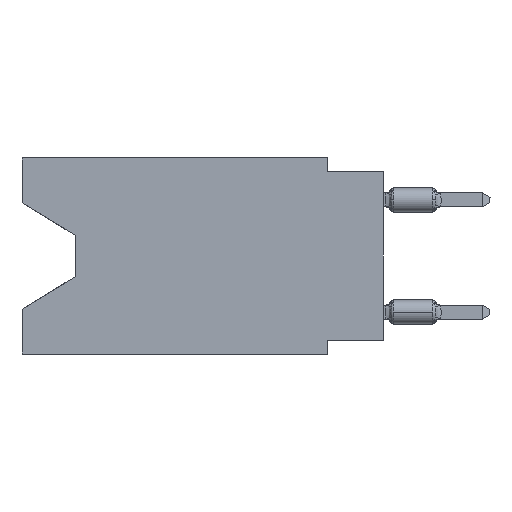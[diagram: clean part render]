
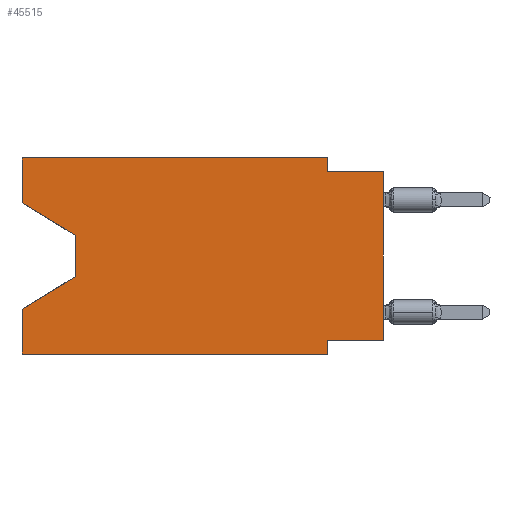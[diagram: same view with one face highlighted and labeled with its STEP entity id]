
A CAD part, left-side view. The second image highlights one B-rep face of the part: STEP entity #45515.
In plain terms, the highlighted planar face has unit normal (-1, 0, 0).
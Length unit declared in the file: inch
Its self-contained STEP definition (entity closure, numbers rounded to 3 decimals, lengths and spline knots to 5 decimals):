
#529 = VERTEX_POINT ( 'NONE', #34901 ) ;
#564 = CARTESIAN_POINT ( 'NONE',  ( 0., 0.645, 0. ) ) ;
#2122 = VECTOR ( 'NONE', #46059, 39.37008 ) ;
#2674 = VERTEX_POINT ( 'NONE', #3748 ) ;
#3398 = DIRECTION ( 'NONE',  ( 0., -0.855, -0.519 ) ) ;
#3622 = ORIENTED_EDGE ( 'NONE', *, *, #26162, .F. ) ;
#3748 = CARTESIAN_POINT ( 'NONE',  ( 0., 0., -0.025 ) ) ;
#3914 = DIRECTION ( 'NONE',  ( 1., 0., 0. ) ) ;
#4079 = DIRECTION ( 'NONE',  ( 0., 0., 1. ) ) ;
#5508 = VERTEX_POINT ( 'NONE', #14268 ) ;
#5778 = CARTESIAN_POINT ( 'NONE',  ( 0., 0.1, -0.325 ) ) ;
#5902 = VERTEX_POINT ( 'NONE', #14208 ) ;
#8015 = CARTESIAN_POINT ( 'NONE',  ( 0., 0., -0.325 ) ) ;
#8222 = ORIENTED_EDGE ( 'NONE', *, *, #21422, .T. ) ;
#8498 = CARTESIAN_POINT ( 'NONE',  ( 0., 0., 0. ) ) ;
#8778 = DIRECTION ( 'NONE',  ( 0., 0.855, -0.519 ) ) ;
#9549 = ORIENTED_EDGE ( 'NONE', *, *, #32910, .F. ) ;
#9821 = EDGE_CURVE ( 'NONE', #33772, #2674, #44464, .T. ) ;
#10688 = ORIENTED_EDGE ( 'NONE', *, *, #47461, .F. ) ;
#11383 = EDGE_LOOP ( 'NONE', ( #43853, #8222, #11428, #39040, #36704, #3622, #36683, #20189, #9549, #22524, #10688, #49818 ) ) ;
#11428 = ORIENTED_EDGE ( 'NONE', *, *, #24532, .T. ) ;
#11602 = VECTOR ( 'NONE', #18971, 39.37008 ) ;
#11731 = DIRECTION ( 'NONE',  ( 0., -1., 0. ) ) ;
#11938 = CARTESIAN_POINT ( 'NONE',  ( 0., 0.55, -0.138 ) ) ;
#11953 = CARTESIAN_POINT ( 'NONE',  ( 0., 0.1, -0.025 ) ) ;
#12722 = CARTESIAN_POINT ( 'NONE',  ( 0., 0.55, -0.212 ) ) ;
#12982 = LINE ( 'NONE', #564, #30357 ) ;
#13359 = VECTOR ( 'NONE', #38359, 39.37008 ) ;
#14208 = CARTESIAN_POINT ( 'NONE',  ( 0., 0.645, -0.26975 ) ) ;
#14226 = EDGE_CURVE ( 'NONE', #33772, #21080, #36258, .T. ) ;
#14268 = CARTESIAN_POINT ( 'NONE',  ( 0., 0.1, -0.35 ) ) ;
#14558 = CARTESIAN_POINT ( 'NONE',  ( 0., 0.645, -0.08025 ) ) ;
#16244 = DIRECTION ( 'NONE',  ( 0., 0., -1. ) ) ;
#18024 = VECTOR ( 'NONE', #38804, 39.37008 ) ;
#18451 = LINE ( 'NONE', #30900, #11602 ) ;
#18971 = DIRECTION ( 'NONE',  ( 0., 0., -1. ) ) ;
#19295 = CARTESIAN_POINT ( 'NONE',  ( 0., 0.645, -0.35 ) ) ;
#20014 = DIRECTION ( 'NONE',  ( 0., 0., -1. ) ) ;
#20102 = PLANE ( 'NONE',  #47299 ) ;
#20189 = ORIENTED_EDGE ( 'NONE', *, *, #9821, .T. ) ;
#20304 = LINE ( 'NONE', #11938, #49593 ) ;
#20643 = FACE_OUTER_BOUND ( 'NONE', #11383, .T. ) ;
#20827 = CARTESIAN_POINT ( 'NONE',  ( 0., 0.1, -0.35 ) ) ;
#21080 = VERTEX_POINT ( 'NONE', #5778 ) ;
#21113 = EDGE_CURVE ( 'NONE', #529, #47254, #25495, .T. ) ;
#21303 = EDGE_CURVE ( 'NONE', #53273, #43360, #18451, .T. ) ;
#21422 = EDGE_CURVE ( 'NONE', #52763, #30456, #20304, .T. ) ;
#21945 = EDGE_CURVE ( 'NONE', #44013, #5508, #42153, .T. ) ;
#22401 = LINE ( 'NONE', #14558, #48359 ) ;
#22524 = ORIENTED_EDGE ( 'NONE', *, *, #21303, .F. ) ;
#22560 = CARTESIAN_POINT ( 'NONE',  ( 0., 0.1, 0. ) ) ;
#24532 = EDGE_CURVE ( 'NONE', #30456, #5902, #49339, .T. ) ;
#25495 = LINE ( 'NONE', #46588, #2122 ) ;
#26162 = EDGE_CURVE ( 'NONE', #21080, #5508, #48696, .T. ) ;
#26742 = VECTOR ( 'NONE', #49594, 39.37008 ) ;
#27888 = VECTOR ( 'NONE', #11731, 39.37008 ) ;
#30357 = VECTOR ( 'NONE', #4079, 39.37008 ) ;
#30456 = VERTEX_POINT ( 'NONE', #12722 ) ;
#30494 = EDGE_CURVE ( 'NONE', #44013, #5902, #12982, .T. ) ;
#30900 = CARTESIAN_POINT ( 'NONE',  ( 0., 0.1, 0. ) ) ;
#32210 = DIRECTION ( 'NONE',  ( 0., 1., 0. ) ) ;
#32302 = CARTESIAN_POINT ( 'NONE',  ( 0., 0.55, -0.212 ) ) ;
#32910 = EDGE_CURVE ( 'NONE', #43360, #2674, #39858, .T. ) ;
#33772 = VERTEX_POINT ( 'NONE', #8015 ) ;
#34450 = VECTOR ( 'NONE', #20014, 39.37008 ) ;
#34901 = CARTESIAN_POINT ( 'NONE',  ( 0., 0.645, -0.08025 ) ) ;
#36258 = LINE ( 'NONE', #52778, #46795 ) ;
#36599 = CARTESIAN_POINT ( 'NONE',  ( 0., 0.645, 0. ) ) ;
#36683 = ORIENTED_EDGE ( 'NONE', *, *, #14226, .F. ) ;
#36704 = ORIENTED_EDGE ( 'NONE', *, *, #21945, .T. ) ;
#38359 = DIRECTION ( 'NONE',  ( 0., -1., 0. ) ) ;
#38804 = DIRECTION ( 'NONE',  ( 0., -1., 0. ) ) ;
#39040 = ORIENTED_EDGE ( 'NONE', *, *, #30494, .F. ) ;
#39858 = LINE ( 'NONE', #45715, #27888 ) ;
#41129 = CARTESIAN_POINT ( 'NONE',  ( 0., 0.55, -0.138 ) ) ;
#42153 = LINE ( 'NONE', #45662, #13359 ) ;
#42598 = CARTESIAN_POINT ( 'NONE',  ( 0., 0.645, 0. ) ) ;
#42874 = CARTESIAN_POINT ( 'NONE',  ( 0., 0.645, 0. ) ) ;
#43360 = VERTEX_POINT ( 'NONE', #11953 ) ;
#43853 = ORIENTED_EDGE ( 'NONE', *, *, #48521, .T. ) ;
#44013 = VERTEX_POINT ( 'NONE', #19295 ) ;
#44464 = LINE ( 'NONE', #8498, #26742 ) ;
#45259 = DIRECTION ( 'NONE',  ( 0., 0., -1. ) ) ;
#45515 = ADVANCED_FACE ( 'NONE', ( #20643 ), #20102, .F. ) ;
#45662 = CARTESIAN_POINT ( 'NONE',  ( 0., 0.645, -0.35 ) ) ;
#45715 = CARTESIAN_POINT ( 'NONE',  ( 0., 0., -0.025 ) ) ;
#46059 = DIRECTION ( 'NONE',  ( 0., 0., 1. ) ) ;
#46410 = VECTOR ( 'NONE', #8778, 39.37008 ) ;
#46588 = CARTESIAN_POINT ( 'NONE',  ( 0., 0.645, 0. ) ) ;
#46795 = VECTOR ( 'NONE', #32210, 39.37008 ) ;
#46914 = LINE ( 'NONE', #42874, #18024 ) ;
#47254 = VERTEX_POINT ( 'NONE', #42598 ) ;
#47299 = AXIS2_PLACEMENT_3D ( 'NONE', #36599, #3914, #45259 ) ;
#47461 = EDGE_CURVE ( 'NONE', #47254, #53273, #46914, .T. ) ;
#48359 = VECTOR ( 'NONE', #3398, 39.37008 ) ;
#48521 = EDGE_CURVE ( 'NONE', #529, #52763, #22401, .T. ) ;
#48696 = LINE ( 'NONE', #20827, #34450 ) ;
#49339 = LINE ( 'NONE', #32302, #46410 ) ;
#49593 = VECTOR ( 'NONE', #16244, 39.37008 ) ;
#49594 = DIRECTION ( 'NONE',  ( 0., 0., 1. ) ) ;
#49818 = ORIENTED_EDGE ( 'NONE', *, *, #21113, .F. ) ;
#52763 = VERTEX_POINT ( 'NONE', #41129 ) ;
#52778 = CARTESIAN_POINT ( 'NONE',  ( 0., 0., -0.325 ) ) ;
#53273 = VERTEX_POINT ( 'NONE', #22560 ) ;
